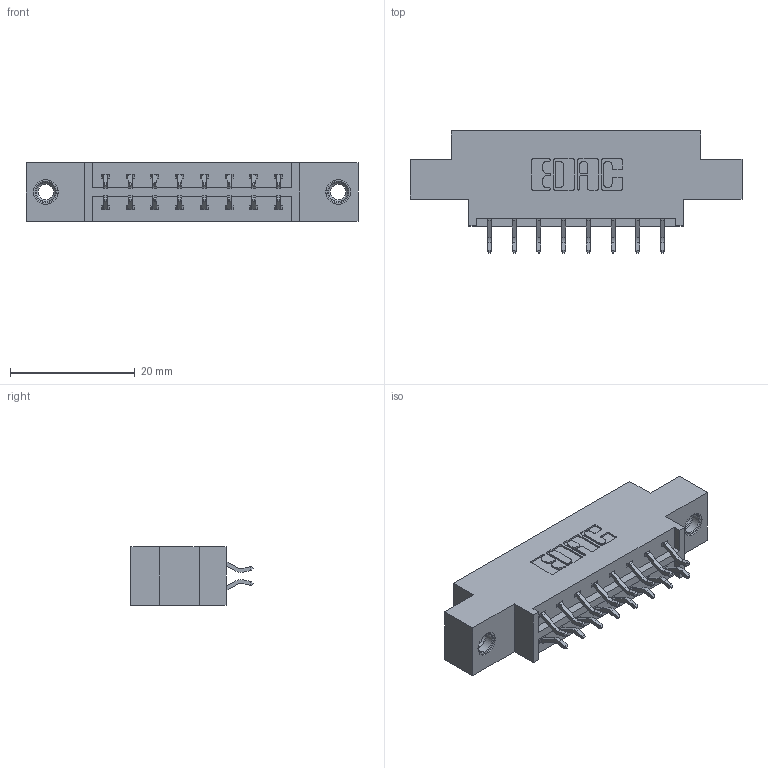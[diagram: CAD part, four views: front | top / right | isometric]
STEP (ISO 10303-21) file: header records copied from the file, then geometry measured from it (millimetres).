
FILE_DESCRIPTION (( 'STEP AP203' ), '1' );
FILE_NAME ('833-016-556-807.STEP', '2020-05-31T18:48:24', ( '' ), ( '' ), 'SwSTEP 2.0', 'SolidWorks 2020', '' );
FILE_SCHEMA (( 'CONFIG_CONTROL_DESIGN' ));
Length unit declared in the file: inch
Products named in the file (4): 833-016-556-807; 833 Part_Offset - .156 Dia - TI; 345-250-001_345-250-005-103; 345-292-001_556 Tail
Assembly tree (19 placements, depth 2):
  833-016-556-807
    833 Part_Offset - .156 Dia - TI
    345-292-001_556 Tail  x16
    345-250-001_345-250-005-103  x2
Bounding box: 53.24 x 19.57 x 9.4 mm (x, y, z)
Volume: 4875.4 mm3; surface area: 5637.8 mm2
Topology: 19 solids, 19 shells, 1106 faces, 3227 edges, 2122 vertices
Faces by surface type: plane 746, cylinder 344, cone 12, torus 4
Entity records: 11082 total; most frequent: CARTESIAN_POINT 1877, ORIENTED_EDGE 1794, DIRECTION 1683, EDGE_CURVE 897, VECTOR 741, LINE 741, VERTEX_POINT 592, AXIS2_PLACEMENT_3D 471
